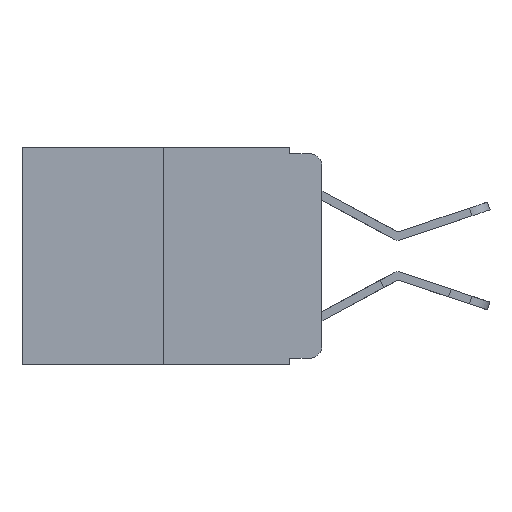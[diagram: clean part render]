
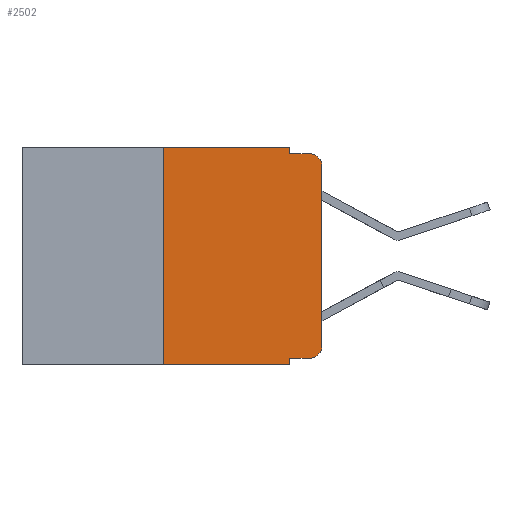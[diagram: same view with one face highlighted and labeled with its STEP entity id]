
A CAD part, left-side view. The second image highlights one B-rep face of the part: STEP entity #2502.
In plain terms, the highlighted planar face has unit normal (-1, 0, 0).
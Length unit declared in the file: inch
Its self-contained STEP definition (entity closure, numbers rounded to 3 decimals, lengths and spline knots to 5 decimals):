
#406 = CARTESIAN_POINT ( 'NONE',  ( 0., 0.25, 0. ) ) ;
#622 = CARTESIAN_POINT ( 'NONE',  ( 0., 0.02, -0.01 ) ) ;
#711 = ORIENTED_EDGE ( 'NONE', *, *, #26561, .T. ) ;
#713 = VERTEX_POINT ( 'NONE', #22295 ) ;
#747 = LINE ( 'NONE', #13566, #7714 ) ;
#1165 = EDGE_CURVE ( 'NONE', #13706, #7188, #26348, .T. ) ;
#1859 = LINE ( 'NONE', #7846, #25192 ) ;
#2099 = ORIENTED_EDGE ( 'NONE', *, *, #14042, .T. ) ;
#2301 = ORIENTED_EDGE ( 'NONE', *, *, #22296, .F. ) ;
#2404 = CARTESIAN_POINT ( 'NONE',  ( 0., 0., -0.313 ) ) ;
#2502 = ADVANCED_FACE ( 'NONE', ( #17984 ), #8545, .F. ) ;
#2905 = VECTOR ( 'NONE', #3921, 39.37008 ) ;
#3420 = ORIENTED_EDGE ( 'NONE', *, *, #12412, .T. ) ;
#3421 = EDGE_CURVE ( 'NONE', #22549, #10804, #16953, .T. ) ;
#3921 = DIRECTION ( 'NONE',  ( 0., 0., -1. ) ) ;
#5022 = DIRECTION ( 'NONE',  ( 0., -1., 0. ) ) ;
#5931 = CARTESIAN_POINT ( 'NONE',  ( 0., 0.02, -0.313 ) ) ;
#6290 = EDGE_CURVE ( 'NONE', #13300, #22549, #21708, .T. ) ;
#6371 = ORIENTED_EDGE ( 'NONE', *, *, #27456, .F. ) ;
#6528 = DIRECTION ( 'NONE',  ( -1., 0., 0. ) ) ;
#6566 = CARTESIAN_POINT ( 'NONE',  ( 0., 0.473, -0.343 ) ) ;
#7188 = VERTEX_POINT ( 'NONE', #622 ) ;
#7714 = VECTOR ( 'NONE', #17754, 39.37008 ) ;
#7846 = CARTESIAN_POINT ( 'NONE',  ( 0., 0.051, -0.333 ) ) ;
#8454 = DIRECTION ( 'NONE',  ( 1., 0., 0. ) ) ;
#8545 = PLANE ( 'NONE',  #15765 ) ;
#8856 = DIRECTION ( 'NONE',  ( 0., 0., -1. ) ) ;
#8994 = VERTEX_POINT ( 'NONE', #15740 ) ;
#10442 = DIRECTION ( 'NONE',  ( -1., 0., 0. ) ) ;
#10804 = VERTEX_POINT ( 'NONE', #13744 ) ;
#11671 = CARTESIAN_POINT ( 'NONE',  ( 0., 0.051, -0.01 ) ) ;
#11746 = ORIENTED_EDGE ( 'NONE', *, *, #19747, .F. ) ;
#11947 = ORIENTED_EDGE ( 'NONE', *, *, #1165, .T. ) ;
#12050 = CARTESIAN_POINT ( 'NONE',  ( 0., 0.25, -0.343 ) ) ;
#12412 = EDGE_CURVE ( 'NONE', #13300, #713, #18269, .T. ) ;
#13300 = VERTEX_POINT ( 'NONE', #12050 ) ;
#13566 = CARTESIAN_POINT ( 'NONE',  ( 0., 0.051, 0. ) ) ;
#13706 = VERTEX_POINT ( 'NONE', #15379 ) ;
#13744 = CARTESIAN_POINT ( 'NONE',  ( 0., 0.051, 0. ) ) ;
#13951 = LINE ( 'NONE', #26267, #26622 ) ;
#14042 = EDGE_CURVE ( 'NONE', #8994, #27501, #1859, .T. ) ;
#14393 = ORIENTED_EDGE ( 'NONE', *, *, #23222, .T. ) ;
#14913 = CARTESIAN_POINT ( 'NONE',  ( 0., 0.02, -0.03 ) ) ;
#15048 = DIRECTION ( 'NONE',  ( 0., 0., 1. ) ) ;
#15379 = CARTESIAN_POINT ( 'NONE',  ( 0., 0., -0.03 ) ) ;
#15468 = DIRECTION ( 'NONE',  ( 0., 0., 1. ) ) ;
#15740 = CARTESIAN_POINT ( 'NONE',  ( 0., 0.051, -0.333 ) ) ;
#15765 = AXIS2_PLACEMENT_3D ( 'NONE', #25161, #8454, #25355 ) ;
#16396 = CARTESIAN_POINT ( 'NONE',  ( 0., 0.02, -0.333 ) ) ;
#16953 = LINE ( 'NONE', #23865, #23295 ) ;
#17703 = VECTOR ( 'NONE', #15048, 39.37008 ) ;
#17754 = DIRECTION ( 'NONE',  ( 0., 0., -1. ) ) ;
#17790 = VERTEX_POINT ( 'NONE', #2404 ) ;
#17984 = FACE_OUTER_BOUND ( 'NONE', #25012, .T. ) ;
#18079 = AXIS2_PLACEMENT_3D ( 'NONE', #5931, #10442, #18829 ) ;
#18269 = LINE ( 'NONE', #6566, #18962 ) ;
#18829 = DIRECTION ( 'NONE',  ( 0., 0., -1. ) ) ;
#18962 = VECTOR ( 'NONE', #21405, 39.37008 ) ;
#19747 = EDGE_CURVE ( 'NONE', #8994, #713, #21218, .T. ) ;
#21218 = LINE ( 'NONE', #25173, #2905 ) ;
#21405 = DIRECTION ( 'NONE',  ( 0., -1., 0. ) ) ;
#21708 = LINE ( 'NONE', #406, #17703 ) ;
#22233 = ORIENTED_EDGE ( 'NONE', *, *, #3421, .F. ) ;
#22295 = CARTESIAN_POINT ( 'NONE',  ( 0., 0.051, -0.343 ) ) ;
#22296 = EDGE_CURVE ( 'NONE', #10804, #24139, #747, .T. ) ;
#22549 = VERTEX_POINT ( 'NONE', #27435 ) ;
#22560 = ORIENTED_EDGE ( 'NONE', *, *, #6290, .F. ) ;
#23222 = EDGE_CURVE ( 'NONE', #27501, #17790, #26755, .T. ) ;
#23226 = AXIS2_PLACEMENT_3D ( 'NONE', #14913, #6528, #8856 ) ;
#23295 = VECTOR ( 'NONE', #5022, 39.37008 ) ;
#23865 = CARTESIAN_POINT ( 'NONE',  ( 0., 0.473, 0. ) ) ;
#24059 = CARTESIAN_POINT ( 'NONE',  ( 0., 0.051, -0.01 ) ) ;
#24139 = VERTEX_POINT ( 'NONE', #11671 ) ;
#24140 = DIRECTION ( 'NONE',  ( 0., -1., 0. ) ) ;
#25012 = EDGE_LOOP ( 'NONE', ( #711, #11947, #6371, #2301, #22233, #22560, #3420, #11746, #2099, #14393 ) ) ;
#25161 = CARTESIAN_POINT ( 'NONE',  ( 0., 0.473, 0. ) ) ;
#25173 = CARTESIAN_POINT ( 'NONE',  ( 0., 0.051, 0. ) ) ;
#25192 = VECTOR ( 'NONE', #26799, 39.37008 ) ;
#25355 = DIRECTION ( 'NONE',  ( 0., 0., -1. ) ) ;
#26267 = CARTESIAN_POINT ( 'NONE',  ( 0., 0., 0. ) ) ;
#26348 = CIRCLE ( 'NONE', #23226, 0.02 ) ;
#26561 = EDGE_CURVE ( 'NONE', #17790, #13706, #13951, .T. ) ;
#26622 = VECTOR ( 'NONE', #15468, 39.37008 ) ;
#26755 = CIRCLE ( 'NONE', #18079, 0.02 ) ;
#26799 = DIRECTION ( 'NONE',  ( 0., -1., 0. ) ) ;
#26868 = LINE ( 'NONE', #24059, #27555 ) ;
#27435 = CARTESIAN_POINT ( 'NONE',  ( 0., 0.25, 0. ) ) ;
#27456 = EDGE_CURVE ( 'NONE', #24139, #7188, #26868, .T. ) ;
#27501 = VERTEX_POINT ( 'NONE', #16396 ) ;
#27555 = VECTOR ( 'NONE', #24140, 39.37008 ) ;
